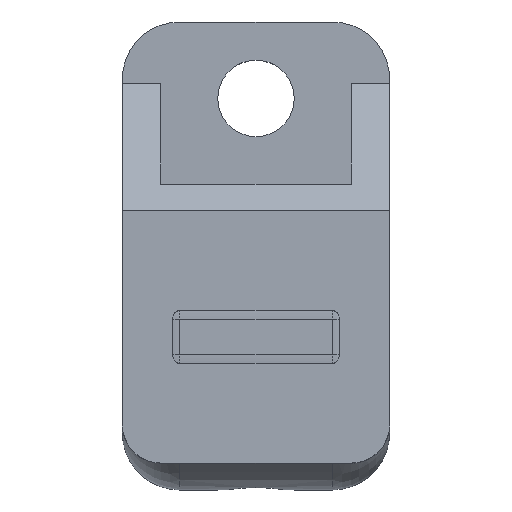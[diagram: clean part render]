
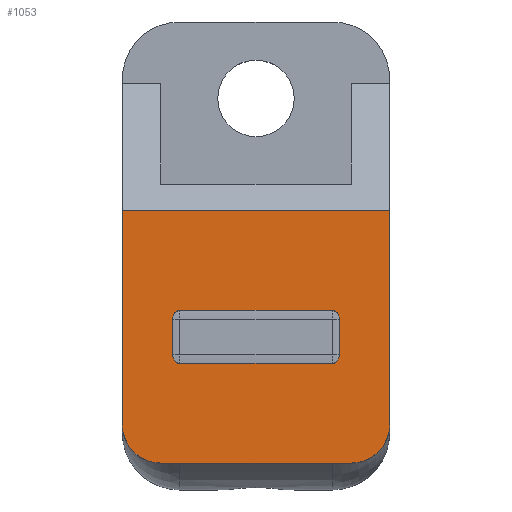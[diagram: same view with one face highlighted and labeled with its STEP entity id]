
A CAD part, top view. The second image highlights one B-rep face of the part: STEP entity #1053.
In plain terms, the highlighted planar face has unit normal (0, 0, 1).
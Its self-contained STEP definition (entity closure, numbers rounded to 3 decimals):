
#10 = CARTESIAN_POINT ( 'NONE',  ( -54.141, -14.919, 27.645 ) ) ;
#17 = LINE ( 'NONE', #3297, #2081 ) ;
#31 = VERTEX_POINT ( 'NONE', #973 ) ;
#70 = EDGE_CURVE ( 'NONE', #2096, #94, #2419, .T. ) ;
#74 = ORIENTED_EDGE ( 'NONE', *, *, #70, .F. ) ;
#94 = VERTEX_POINT ( 'NONE', #2425 ) ;
#134 = CARTESIAN_POINT ( 'NONE',  ( -58.35, -12.138, 27.645 ) ) ;
#138 = FACE_BOUND ( 'NONE', #2137, .T. ) ;
#152 = CARTESIAN_POINT ( 'NONE',  ( -53.993, -21.529, 27.645 ) ) ;
#201 = VERTEX_POINT ( 'NONE', #2663 ) ;
#229 = CARTESIAN_POINT ( 'NONE',  ( -62.35, -14.919, 27.645 ) ) ;
#261 = VERTEX_POINT ( 'NONE', #388 ) ;
#272 = CARTESIAN_POINT ( 'NONE',  ( -62.35, -12.138, 27.645 ) ) ;
#317 = EDGE_CURVE ( 'NONE', #2184, #2420, #3451, .T. ) ;
#388 = CARTESIAN_POINT ( 'NONE',  ( -62.35, -14.919, 27.645 ) ) ;
#430 = ORIENTED_EDGE ( 'NONE', *, *, #2952, .F. ) ;
#576 =( BOUNDED_CURVE ( )  B_SPLINE_CURVE ( 3, ( #3762, #3776, #2012, #1145 ),
 .UNSPECIFIED., .F., .T. ) 
 B_SPLINE_CURVE_WITH_KNOTS ( ( 4, 4 ),
 ( 3.138, 4.706 ),
 .UNSPECIFIED. ) 
 CURVE ( )  GEOMETRIC_REPRESENTATION_ITEM ( )  RATIONAL_B_SPLINE_CURVE ( ( 1., 0.805, 0.805, 1. ) ) 
 REPRESENTATION_ITEM ( '' )  );
#627 = ORIENTED_EDGE ( 'NONE', *, *, #864, .T. ) ;
#628 =( BOUNDED_CURVE ( )  B_SPLINE_CURVE ( 3, ( #3193, #10, #1432, #2942 ),
 .UNSPECIFIED., .F., .T. ) 
 B_SPLINE_CURVE_WITH_KNOTS ( ( 4, 4 ),
 ( 6.279, 7.847 ),
 .UNSPECIFIED. ) 
 CURVE ( )  GEOMETRIC_REPRESENTATION_ITEM ( )  RATIONAL_B_SPLINE_CURVE ( ( 1., 0.805, 0.805, 1. ) ) 
 REPRESENTATION_ITEM ( '' )  );
#722 = CARTESIAN_POINT ( 'NONE',  ( -53.993, -12.6, 27.645 ) ) ;
#757 = PLANE ( 'NONE',  #2113 ) ;
#779 = EDGE_CURVE ( 'NONE', #94, #1128, #3313, .T. ) ;
#806 = VERTEX_POINT ( 'NONE', #1137 ) ;
#853 = ORIENTED_EDGE ( 'NONE', *, *, #1987, .F. ) ;
#861 = EDGE_CURVE ( 'NONE', #806, #201, #628, .T. ) ;
#864 = EDGE_CURVE ( 'NONE', #2096, #2184, #2219, .T. ) ;
#933 = FACE_OUTER_BOUND ( 'NONE', #1698, .T. ) ;
#973 = CARTESIAN_POINT ( 'NONE',  ( -62.708, -12.6, 27.645 ) ) ;
#986 = VECTOR ( 'NONE', #3607, 1000. ) ;
#1053 = ADVANCED_FACE ( 'NONE', ( #933, #138 ), #757, .F. ) ;
#1072 = CARTESIAN_POINT ( 'NONE',  ( -65.35, -20.13, 27.645 ) ) ;
#1122 = CARTESIAN_POINT ( 'NONE',  ( -51.35, -20.13, 27.645 ) ) ;
#1128 = VERTEX_POINT ( 'NONE', #1879 ) ;
#1137 = CARTESIAN_POINT ( 'NONE',  ( -54.35, -14.919, 27.645 ) ) ;
#1145 = CARTESIAN_POINT ( 'NONE',  ( -62.708, -12.6, 27.645 ) ) ;
#1156 = DIRECTION ( 'NONE',  ( 0., 1., 0. ) ) ;
#1225 = EDGE_CURVE ( 'NONE', #3275, #31, #17, .T. ) ;
#1227 = ORIENTED_EDGE ( 'NONE', *, *, #3259, .T. ) ;
#1251 = DIRECTION ( 'NONE',  ( 0., -1., 0. ) ) ;
#1323 = CARTESIAN_POINT ( 'NONE',  ( -54.35, -12.138, 27.645 ) ) ;
#1367 = VERTEX_POINT ( 'NONE', #3162 ) ;
#1398 = CARTESIAN_POINT ( 'NONE',  ( -62.708, -14.728, 27.645 ) ) ;
#1415 = VERTEX_POINT ( 'NONE', #722 ) ;
#1428 = CARTESIAN_POINT ( 'NONE',  ( -62.708, -14.458, 27.645 ) ) ;
#1432 = CARTESIAN_POINT ( 'NONE',  ( -53.993, -14.728, 27.645 ) ) ;
#1437 = CARTESIAN_POINT ( 'NONE',  ( -62.708, -14.458, 27.645 ) ) ;
#1446 = VECTOR ( 'NONE', #2616, 1000. ) ;
#1465 = EDGE_CURVE ( 'NONE', #1367, #2384, #3083, .T. ) ;
#1493 = DIRECTION ( 'NONE',  ( 0., 0., -1. ) ) ;
#1565 = EDGE_CURVE ( 'NONE', #806, #261, #2364, .T. ) ;
#1678 = ORIENTED_EDGE ( 'NONE', *, *, #779, .F. ) ;
#1698 = EDGE_LOOP ( 'NONE', ( #1678, #74, #627, #3327, #1814, #3568 ) ) ;
#1814 = ORIENTED_EDGE ( 'NONE', *, *, #1878, .F. ) ;
#1826 = ORIENTED_EDGE ( 'NONE', *, *, #1465, .F. ) ;
#1829 = DIRECTION ( 'NONE',  ( 0., 0., -1. ) ) ;
#1834 = ORIENTED_EDGE ( 'NONE', *, *, #2602, .T. ) ;
#1878 = EDGE_CURVE ( 'NONE', #3380, #2420, #3050, .T. ) ;
#1879 = CARTESIAN_POINT ( 'NONE',  ( -63.35, -20.13, 27.645 ) ) ;
#1919 = DIRECTION ( 'NONE',  ( -1., 0., 0. ) ) ;
#1941 = AXIS2_PLACEMENT_3D ( 'NONE', #2121, #1829, #1251 ) ;
#1943 = LINE ( 'NONE', #152, #2544 ) ;
#1987 = EDGE_CURVE ( 'NONE', #2384, #31, #576, .T. ) ;
#2012 = CARTESIAN_POINT ( 'NONE',  ( -62.708, -12.329, 27.645 ) ) ;
#2034 = CIRCLE ( 'NONE', #2989, 2. ) ;
#2072 = EDGE_CURVE ( 'NONE', #1128, #3380, #2034, .T. ) ;
#2076 = ORIENTED_EDGE ( 'NONE', *, *, #861, .F. ) ;
#2081 = VECTOR ( 'NONE', #2124, 1000. ) ;
#2096 = VERTEX_POINT ( 'NONE', #3244 ) ;
#2113 = AXIS2_PLACEMENT_3D ( 'NONE', #2805, #3104, #3398 ) ;
#2121 = CARTESIAN_POINT ( 'NONE',  ( -53.35, -18.13, 27.645 ) ) ;
#2124 = DIRECTION ( 'NONE',  ( 0., 1., 0. ) ) ;
#2137 = EDGE_LOOP ( 'NONE', ( #1834, #430, #2076, #3069, #1227, #2339, #853, #1826 ) ) ;
#2184 = VERTEX_POINT ( 'NONE', #3615 ) ;
#2191 = CARTESIAN_POINT ( 'NONE',  ( -53.993, -12.329, 27.645 ) ) ;
#2200 = CARTESIAN_POINT ( 'NONE',  ( -54.141, -12.138, 27.645 ) ) ;
#2219 = LINE ( 'NONE', #3507, #1446 ) ;
#2315 = VECTOR ( 'NONE', #3370, 1000. ) ;
#2339 = ORIENTED_EDGE ( 'NONE', *, *, #1225, .T. ) ;
#2364 = LINE ( 'NONE', #3372, #2739 ) ;
#2384 = VERTEX_POINT ( 'NONE', #272 ) ;
#2419 = CIRCLE ( 'NONE', #1941, 2. ) ;
#2420 = VERTEX_POINT ( 'NONE', #2699 ) ;
#2425 = CARTESIAN_POINT ( 'NONE',  ( -53.35, -20.13, 27.645 ) ) ;
#2544 = VECTOR ( 'NONE', #2853, 1000. ) ;
#2550 = VECTOR ( 'NONE', #3462, 1000. ) ;
#2602 = EDGE_CURVE ( 'NONE', #1367, #1415, #2904, .T. ) ;
#2616 = DIRECTION ( 'NONE',  ( 0., 1., 0. ) ) ;
#2622 =( BOUNDED_CURVE ( )  B_SPLINE_CURVE ( 3, ( #229, #3465, #1398, #1428 ),
 .UNSPECIFIED., .F., .F. ) 
 B_SPLINE_CURVE_WITH_KNOTS ( ( 4, 4 ),
 ( 3.138, 4.706 ),
 .UNSPECIFIED. ) 
 CURVE ( )  GEOMETRIC_REPRESENTATION_ITEM ( )  RATIONAL_B_SPLINE_CURVE ( ( 1., 0.805, 0.805, 1. ) ) 
 REPRESENTATION_ITEM ( '' )  );
#2663 = CARTESIAN_POINT ( 'NONE',  ( -53.993, -14.458, 27.645 ) ) ;
#2699 = CARTESIAN_POINT ( 'NONE',  ( -65.35, -6.91, 27.645 ) ) ;
#2702 = DIRECTION ( 'NONE',  ( 0., -1., 0. ) ) ;
#2725 = CARTESIAN_POINT ( 'NONE',  ( -51.35, -6.91, 27.645 ) ) ;
#2739 = VECTOR ( 'NONE', #1919, 1000. ) ;
#2805 = CARTESIAN_POINT ( 'NONE',  ( -51.35, -20.13, 27.645 ) ) ;
#2853 = DIRECTION ( 'NONE',  ( 0., 1., 0. ) ) ;
#2904 =( BOUNDED_CURVE ( )  B_SPLINE_CURVE ( 3, ( #1323, #2200, #2191, #3651 ),
 .UNSPECIFIED., .F., .T. ) 
 B_SPLINE_CURVE_WITH_KNOTS ( ( 4, 4 ),
 ( 6.279, 7.847 ),
 .UNSPECIFIED. ) 
 CURVE ( )  GEOMETRIC_REPRESENTATION_ITEM ( )  RATIONAL_B_SPLINE_CURVE ( ( 1., 0.805, 0.805, 1. ) ) 
 REPRESENTATION_ITEM ( '' )  );
#2942 = CARTESIAN_POINT ( 'NONE',  ( -53.993, -14.458, 27.645 ) ) ;
#2952 = EDGE_CURVE ( 'NONE', #201, #1415, #1943, .T. ) ;
#2984 = CARTESIAN_POINT ( 'NONE',  ( -65.35, -18.13, 27.645 ) ) ;
#2989 = AXIS2_PLACEMENT_3D ( 'NONE', #3233, #1493, #2702 ) ;
#3050 = LINE ( 'NONE', #1072, #3136 ) ;
#3069 = ORIENTED_EDGE ( 'NONE', *, *, #1565, .T. ) ;
#3083 = LINE ( 'NONE', #134, #2315 ) ;
#3104 = DIRECTION ( 'NONE',  ( 0., 0., -1. ) ) ;
#3136 = VECTOR ( 'NONE', #1156, 1000. ) ;
#3162 = CARTESIAN_POINT ( 'NONE',  ( -54.35, -12.138, 27.645 ) ) ;
#3193 = CARTESIAN_POINT ( 'NONE',  ( -54.35, -14.919, 27.645 ) ) ;
#3233 = CARTESIAN_POINT ( 'NONE',  ( -63.35, -18.13, 27.645 ) ) ;
#3244 = CARTESIAN_POINT ( 'NONE',  ( -51.35, -18.13, 27.645 ) ) ;
#3259 = EDGE_CURVE ( 'NONE', #261, #3275, #2622, .T. ) ;
#3275 = VERTEX_POINT ( 'NONE', #1437 ) ;
#3297 = CARTESIAN_POINT ( 'NONE',  ( -62.708, -21.529, 27.645 ) ) ;
#3313 = LINE ( 'NONE', #1122, #2550 ) ;
#3327 = ORIENTED_EDGE ( 'NONE', *, *, #317, .T. ) ;
#3370 = DIRECTION ( 'NONE',  ( -1., 0., 0. ) ) ;
#3372 = CARTESIAN_POINT ( 'NONE',  ( -58.35, -14.919, 27.645 ) ) ;
#3380 = VERTEX_POINT ( 'NONE', #2984 ) ;
#3398 = DIRECTION ( 'NONE',  ( 0., 1., 0. ) ) ;
#3451 = LINE ( 'NONE', #2725, #986 ) ;
#3462 = DIRECTION ( 'NONE',  ( -1., 0., 0. ) ) ;
#3465 = CARTESIAN_POINT ( 'NONE',  ( -62.56, -14.919, 27.645 ) ) ;
#3507 = CARTESIAN_POINT ( 'NONE',  ( -51.35, -20.13, 27.645 ) ) ;
#3568 = ORIENTED_EDGE ( 'NONE', *, *, #2072, .F. ) ;
#3607 = DIRECTION ( 'NONE',  ( -1., 0., 0. ) ) ;
#3615 = CARTESIAN_POINT ( 'NONE',  ( -51.35, -6.91, 27.645 ) ) ;
#3651 = CARTESIAN_POINT ( 'NONE',  ( -53.993, -12.6, 27.645 ) ) ;
#3762 = CARTESIAN_POINT ( 'NONE',  ( -62.35, -12.138, 27.645 ) ) ;
#3776 = CARTESIAN_POINT ( 'NONE',  ( -62.56, -12.138, 27.645 ) ) ;
